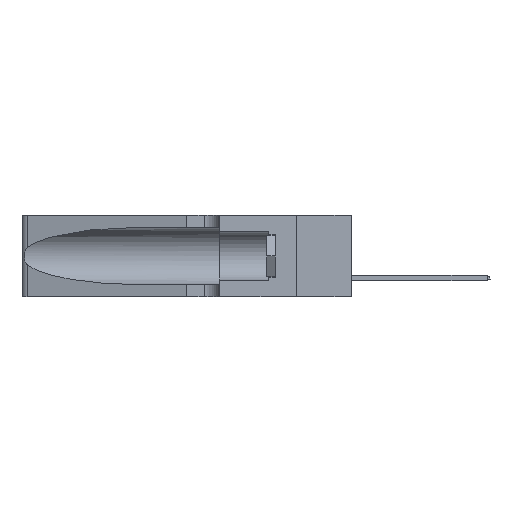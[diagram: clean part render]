
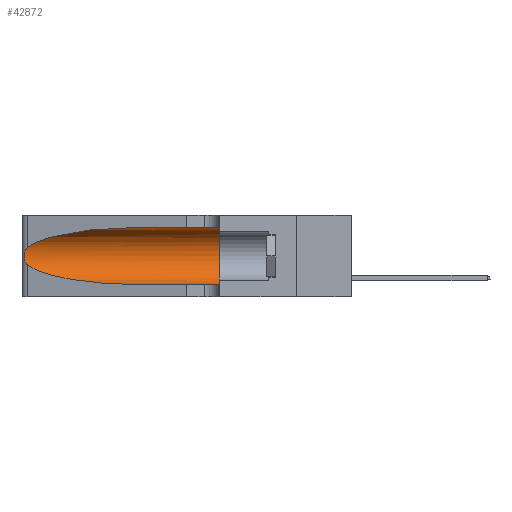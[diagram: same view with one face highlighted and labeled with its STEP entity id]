
A CAD part, left-side view. The second image highlights one B-rep face of the part: STEP entity #42872.
In plain terms, the highlighted cylindrical face has radius 3.308 mm (diameter 6.617 mm), a partial arc.
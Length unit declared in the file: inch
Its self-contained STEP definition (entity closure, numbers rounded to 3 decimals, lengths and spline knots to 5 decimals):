
#248 = FACE_OUTER_BOUND ( 'NONE', #14357, .T. ) ;
#460 = DIRECTION ( 'NONE',  ( 0., 1., 0. ) ) ;
#2090 = B_SPLINE_CURVE_WITH_KNOTS ( 'NONE', 3,
 ( #22211, #25727, #22511, #26049, #36643, #15594, #9512, #33608, #44249, #22802, #37273, #26690, #30362, #33918 ),
 .UNSPECIFIED., .F., .F.,
 ( 4, 2, 2, 2, 2, 2, 4 ),
 ( 0., 0.00027, 0.00053, 0.00107, 0.0016, 0.00187, 0.00214 ),
 .UNSPECIFIED. ) ;
#2704 = CARTESIAN_POINT ( 'NONE',  ( 0.1305, 0.35, 0.31525 ) ) ;
#8800 = CARTESIAN_POINT ( 'NONE',  ( 0.18966, 0.96281, 0.05475 ) ) ;
#8957 = CARTESIAN_POINT ( 'NONE',  ( 0.1305, 0.72297, 0.05475 ) ) ;
#9512 = CARTESIAN_POINT ( 'NONE',  ( 0.26075, 1.23896, 0.19203 ) ) ;
#10326 = ORIENTED_EDGE ( 'NONE', *, *, #12119, .T. ) ;
#11341 = DIRECTION ( 'NONE',  ( 0., 0., 1. ) ) ;
#12119 = EDGE_CURVE ( 'NONE', #42170, #29803, #34523, .T. ) ;
#12747 = ORIENTED_EDGE ( 'NONE', *, *, #27102, .F. ) ;
#13487 = DIRECTION ( 'NONE',  ( 0., -1., 0. ) ) ;
#13574 = VERTEX_POINT ( 'NONE', #2704 ) ;
#14357 = EDGE_LOOP ( 'NONE', ( #10326, #21777, #18002, #16262, #17702, #12747 ) ) ;
#14378 = EDGE_CURVE ( 'NONE', #29803, #22386, #2090, .T. ) ;
#15539 = VERTEX_POINT ( 'NONE', #30820 ) ;
#15594 = CARTESIAN_POINT ( 'NONE',  ( 0.26018, 1.23835, 0.19895 ) ) ;
#16262 = ORIENTED_EDGE ( 'NONE', *, *, #43290, .T. ) ;
#16428 = AXIS2_PLACEMENT_3D ( 'NONE', #17453, #35396, #38962 ) ;
#17453 = CARTESIAN_POINT ( 'NONE',  ( 0.1305, 1.61858, 0.185 ) ) ;
#17549 =( BOUNDED_CURVE ( )  B_SPLINE_CURVE ( 3, ( #42747, #29848, #8800, #8957 ),
 .UNSPECIFIED., .F., .F. ) 
 B_SPLINE_CURVE_WITH_KNOTS ( ( 4, 4 ),
 ( 3.44316, 4.71239 ),
 .UNSPECIFIED. ) 
 CURVE ( )  GEOMETRIC_REPRESENTATION_ITEM ( )  RATIONAL_B_SPLINE_CURVE ( ( 1., 0.87, 0.87, 1. ) ) 
 REPRESENTATION_ITEM ( '' )  );
#17702 = ORIENTED_EDGE ( 'NONE', *, *, #29181, .F. ) ;
#18002 = ORIENTED_EDGE ( 'NONE', *, *, #31193, .T. ) ;
#21690 = CARTESIAN_POINT ( 'NONE',  ( 0.1305, 0.72297, 0.31525 ) ) ;
#21777 = ORIENTED_EDGE ( 'NONE', *, *, #14378, .T. ) ;
#22211 = CARTESIAN_POINT ( 'NONE',  ( 0.25487, 1.22718, 0.22369 ) ) ;
#22353 = LINE ( 'NONE', #25400, #44970 ) ;
#22386 = VERTEX_POINT ( 'NONE', #40980 ) ;
#22511 = CARTESIAN_POINT ( 'NONE',  ( 0.25639, 1.23184, 0.21858 ) ) ;
#22774 = CYLINDRICAL_SURFACE ( 'NONE', #16428, 0.13025 ) ;
#22802 = CARTESIAN_POINT ( 'NONE',  ( 0.25856, 1.23593, 0.16098 ) ) ;
#23267 = CARTESIAN_POINT ( 'NONE',  ( 0.1305, 0.72297, 0.31525 ) ) ;
#23890 = LINE ( 'NONE', #37910, #34361 ) ;
#25400 = CARTESIAN_POINT ( 'NONE',  ( 0.1305, 1.61858, 0.31525 ) ) ;
#25727 = CARTESIAN_POINT ( 'NONE',  ( 0.25555, 1.22994, 0.2215 ) ) ;
#26049 = CARTESIAN_POINT ( 'NONE',  ( 0.25787, 1.23484, 0.2124 ) ) ;
#26174 = CARTESIAN_POINT ( 'NONE',  ( 0.18966, 0.96281, 0.31525 ) ) ;
#26468 = AXIS2_PLACEMENT_3D ( 'NONE', #39823, #460, #11341 ) ;
#26690 = CARTESIAN_POINT ( 'NONE',  ( 0.25639, 1.23186, 0.15144 ) ) ;
#27102 = EDGE_CURVE ( 'NONE', #42170, #13574, #22353, .T. ) ;
#29181 = EDGE_CURVE ( 'NONE', #13574, #36005, #39455, .T. ) ;
#29803 = VERTEX_POINT ( 'NONE', #45261 ) ;
#29848 = CARTESIAN_POINT ( 'NONE',  ( 0.2373, 1.15595, 0.08982 ) ) ;
#30035 = DIRECTION ( 'NONE',  ( 0., -1., 0. ) ) ;
#30362 = CARTESIAN_POINT ( 'NONE',  ( 0.25555, 1.22993, 0.14849 ) ) ;
#30820 = CARTESIAN_POINT ( 'NONE',  ( 0.1305, 0.72297, 0.05475 ) ) ;
#31193 = EDGE_CURVE ( 'NONE', #22386, #15539, #17549, .T. ) ;
#32124 = CARTESIAN_POINT ( 'NONE',  ( 0.1305, 0.35, 0.05475 ) ) ;
#33608 = CARTESIAN_POINT ( 'NONE',  ( 0.26075, 1.23896, 0.178 ) ) ;
#33893 = CARTESIAN_POINT ( 'NONE',  ( 0.2373, 1.15595, 0.28018 ) ) ;
#33918 = CARTESIAN_POINT ( 'NONE',  ( 0.25487, 1.22718, 0.14631 ) ) ;
#34361 = VECTOR ( 'NONE', #13487, 39.37008 ) ;
#34523 =( BOUNDED_CURVE ( )  B_SPLINE_CURVE ( 3, ( #23267, #26174, #33893, #44048 ),
 .UNSPECIFIED., .F., .F. ) 
 B_SPLINE_CURVE_WITH_KNOTS ( ( 4, 4 ),
 ( 1.5708, 2.84003 ),
 .UNSPECIFIED. ) 
 CURVE ( )  GEOMETRIC_REPRESENTATION_ITEM ( )  RATIONAL_B_SPLINE_CURVE ( ( 1., 0.87, 0.87, 1. ) ) 
 REPRESENTATION_ITEM ( '' )  );
#35396 = DIRECTION ( 'NONE',  ( 0., -1., 0. ) ) ;
#36005 = VERTEX_POINT ( 'NONE', #32124 ) ;
#36643 = CARTESIAN_POINT ( 'NONE',  ( 0.25854, 1.2359, 0.20912 ) ) ;
#37273 = CARTESIAN_POINT ( 'NONE',  ( 0.25789, 1.23486, 0.15765 ) ) ;
#37910 = CARTESIAN_POINT ( 'NONE',  ( 0.1305, 1.61858, 0.05475 ) ) ;
#38962 = DIRECTION ( 'NONE',  ( 0., 0., -1. ) ) ;
#39455 = CIRCLE ( 'NONE', #26468, 0.13025 ) ;
#39823 = CARTESIAN_POINT ( 'NONE',  ( 0.1305, 0.35, 0.185 ) ) ;
#40980 = CARTESIAN_POINT ( 'NONE',  ( 0.25487, 1.22718, 0.14631 ) ) ;
#42170 = VERTEX_POINT ( 'NONE', #21690 ) ;
#42747 = CARTESIAN_POINT ( 'NONE',  ( 0.25487, 1.22718, 0.14631 ) ) ;
#42872 = ADVANCED_FACE ( 'NONE', ( #248 ), #22774, .F. ) ;
#43290 = EDGE_CURVE ( 'NONE', #15539, #36005, #23890, .T. ) ;
#44048 = CARTESIAN_POINT ( 'NONE',  ( 0.25487, 1.22718, 0.22369 ) ) ;
#44249 = CARTESIAN_POINT ( 'NONE',  ( 0.26017, 1.23833, 0.17102 ) ) ;
#44970 = VECTOR ( 'NONE', #30035, 39.37008 ) ;
#45261 = CARTESIAN_POINT ( 'NONE',  ( 0.25487, 1.22718, 0.22369 ) ) ;
